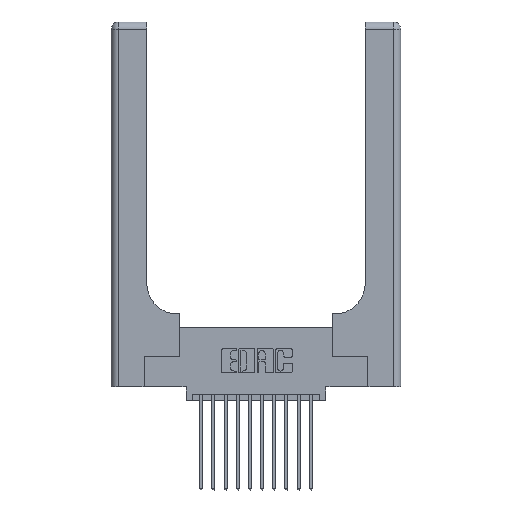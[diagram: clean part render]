
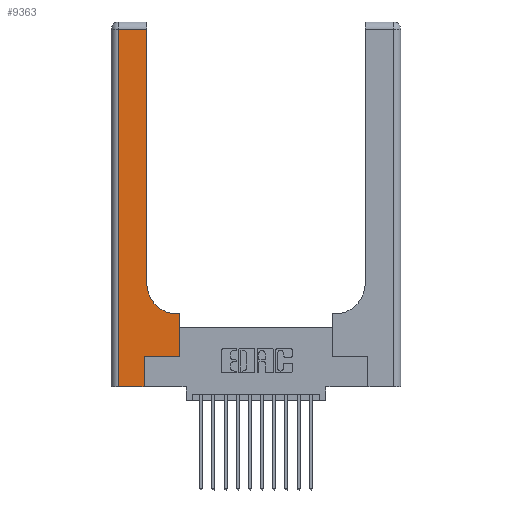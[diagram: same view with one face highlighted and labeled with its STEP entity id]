
A CAD part, top view. The second image highlights one B-rep face of the part: STEP entity #9363.
In plain terms, the highlighted planar face has unit normal (0, 0, 1).
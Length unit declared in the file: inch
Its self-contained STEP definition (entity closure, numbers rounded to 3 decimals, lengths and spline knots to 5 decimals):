
#43 = EDGE_LOOP ( 'NONE', ( #9674, #2728, #7859, #14053, #16846, #5774, #14299, #13248, #6565 ) ) ;
#720 = FACE_OUTER_BOUND ( 'NONE', #43, .T. ) ;
#789 = DIRECTION ( 'NONE',  ( 1., 0., 0. ) ) ;
#917 = DIRECTION ( 'NONE',  ( -1., 0., 0. ) ) ;
#1029 = VECTOR ( 'NONE', #10950, 39.37008 ) ;
#1809 = DIRECTION ( 'NONE',  ( 0., 0., -1. ) ) ;
#2041 = LINE ( 'NONE', #3045, #2475 ) ;
#2226 = CARTESIAN_POINT ( 'NONE',  ( 0., 2.94, 0.37 ) ) ;
#2313 = DIRECTION ( 'NONE',  ( 1., 0., 0. ) ) ;
#2367 = CARTESIAN_POINT ( 'NONE',  ( 0.5585, 0.25, 0.37 ) ) ;
#2475 = VECTOR ( 'NONE', #5865, 39.37008 ) ;
#2570 = VECTOR ( 'NONE', #17037, 39.37008 ) ;
#2728 = ORIENTED_EDGE ( 'NONE', *, *, #13967, .T. ) ;
#3045 = CARTESIAN_POINT ( 'NONE',  ( 0.06, 3., 0.37 ) ) ;
#3140 = VERTEX_POINT ( 'NONE', #12077 ) ;
#3453 = LINE ( 'NONE', #3634, #2570 ) ;
#3634 = CARTESIAN_POINT ( 'NONE',  ( 0.2915, 3., 0.37 ) ) ;
#3696 = PLANE ( 'NONE',  #13719 ) ;
#3764 = EDGE_CURVE ( 'NONE', #3140, #3868, #10428, .T. ) ;
#3822 = CARTESIAN_POINT ( 'NONE',  ( 0.06, 0., 0.37 ) ) ;
#3868 = VERTEX_POINT ( 'NONE', #10648 ) ;
#4468 = VERTEX_POINT ( 'NONE', #5396 ) ;
#4609 = AXIS2_PLACEMENT_3D ( 'NONE', #10109, #1809, #11486 ) ;
#5153 = EDGE_CURVE ( 'NONE', #12816, #16730, #15480, .T. ) ;
#5396 = CARTESIAN_POINT ( 'NONE',  ( 0.06, 2.94, 0.37 ) ) ;
#5606 = CIRCLE ( 'NONE', #4609, 0.25 ) ;
#5738 = LINE ( 'NONE', #7744, #15958 ) ;
#5774 = ORIENTED_EDGE ( 'NONE', *, *, #15898, .T. ) ;
#5865 = DIRECTION ( 'NONE',  ( 0., -1., 0. ) ) ;
#6565 = ORIENTED_EDGE ( 'NONE', *, *, #6595, .T. ) ;
#6595 = EDGE_CURVE ( 'NONE', #14636, #14796, #5606, .T. ) ;
#6719 = LINE ( 'NONE', #2226, #9919 ) ;
#6861 = CARTESIAN_POINT ( 'NONE',  ( 0.2915, 0.6, 0.37 ) ) ;
#7014 = EDGE_CURVE ( 'NONE', #16730, #14636, #17026, .T. ) ;
#7744 = CARTESIAN_POINT ( 'NONE',  ( 0., 0., 0.37 ) ) ;
#7810 = DIRECTION ( 'NONE',  ( -1., 0., 0. ) ) ;
#7859 = ORIENTED_EDGE ( 'NONE', *, *, #16141, .T. ) ;
#8553 = VECTOR ( 'NONE', #2313, 39.37008 ) ;
#8699 = CARTESIAN_POINT ( 'NONE',  ( 0.2915, 2.94, 0.37 ) ) ;
#9228 = DIRECTION ( 'NONE',  ( 0., 0., -1. ) ) ;
#9285 = EDGE_CURVE ( 'NONE', #9402, #3140, #5738, .T. ) ;
#9363 = ADVANCED_FACE ( 'NONE', ( #720 ), #3696, .F. ) ;
#9402 = VERTEX_POINT ( 'NONE', #3822 ) ;
#9452 = CARTESIAN_POINT ( 'NONE',  ( 0.5415, 0.6, 0.37 ) ) ;
#9614 = DIRECTION ( 'NONE',  ( -1., 0., 0. ) ) ;
#9674 = ORIENTED_EDGE ( 'NONE', *, *, #13981, .T. ) ;
#9919 = VECTOR ( 'NONE', #7810, 39.37008 ) ;
#10109 = CARTESIAN_POINT ( 'NONE',  ( 0.5415, 0.85, 0.37 ) ) ;
#10428 = LINE ( 'NONE', #14418, #17339 ) ;
#10648 = CARTESIAN_POINT ( 'NONE',  ( 0.269, 0.25, 0.37 ) ) ;
#10950 = DIRECTION ( 'NONE',  ( 0., 1., 0. ) ) ;
#11486 = DIRECTION ( 'NONE',  ( 1., 0., 0. ) ) ;
#12077 = CARTESIAN_POINT ( 'NONE',  ( 0.269, 0., 0.37 ) ) ;
#12816 = VERTEX_POINT ( 'NONE', #2367 ) ;
#13248 = ORIENTED_EDGE ( 'NONE', *, *, #7014, .T. ) ;
#13315 = CARTESIAN_POINT ( 'NONE',  ( 0.269, 0.25, 0.37 ) ) ;
#13617 = VECTOR ( 'NONE', #9614, 39.37008 ) ;
#13719 = AXIS2_PLACEMENT_3D ( 'NONE', #14512, #9228, #917 ) ;
#13789 = VERTEX_POINT ( 'NONE', #8699 ) ;
#13856 = CARTESIAN_POINT ( 'NONE',  ( 0.5585, 0.6, 0.37 ) ) ;
#13967 = EDGE_CURVE ( 'NONE', #13789, #4468, #6719, .T. ) ;
#13981 = EDGE_CURVE ( 'NONE', #14796, #13789, #3453, .T. ) ;
#14053 = ORIENTED_EDGE ( 'NONE', *, *, #9285, .T. ) ;
#14299 = ORIENTED_EDGE ( 'NONE', *, *, #5153, .T. ) ;
#14418 = CARTESIAN_POINT ( 'NONE',  ( 0.269, 0., 0.37 ) ) ;
#14512 = CARTESIAN_POINT ( 'NONE',  ( 0., 3., 0.37 ) ) ;
#14636 = VERTEX_POINT ( 'NONE', #9452 ) ;
#14796 = VERTEX_POINT ( 'NONE', #15274 ) ;
#15274 = CARTESIAN_POINT ( 'NONE',  ( 0.2915, 0.85, 0.37 ) ) ;
#15480 = LINE ( 'NONE', #17389, #1029 ) ;
#15605 = LINE ( 'NONE', #13315, #8553 ) ;
#15706 = DIRECTION ( 'NONE',  ( 0., 1., 0. ) ) ;
#15898 = EDGE_CURVE ( 'NONE', #3868, #12816, #15605, .T. ) ;
#15958 = VECTOR ( 'NONE', #789, 39.37008 ) ;
#16141 = EDGE_CURVE ( 'NONE', #4468, #9402, #2041, .T. ) ;
#16730 = VERTEX_POINT ( 'NONE', #13856 ) ;
#16846 = ORIENTED_EDGE ( 'NONE', *, *, #3764, .T. ) ;
#17026 = LINE ( 'NONE', #6861, #13617 ) ;
#17037 = DIRECTION ( 'NONE',  ( 0., 1., 0. ) ) ;
#17339 = VECTOR ( 'NONE', #15706, 39.37008 ) ;
#17389 = CARTESIAN_POINT ( 'NONE',  ( 0.5585, 0.25, 0.37 ) ) ;
